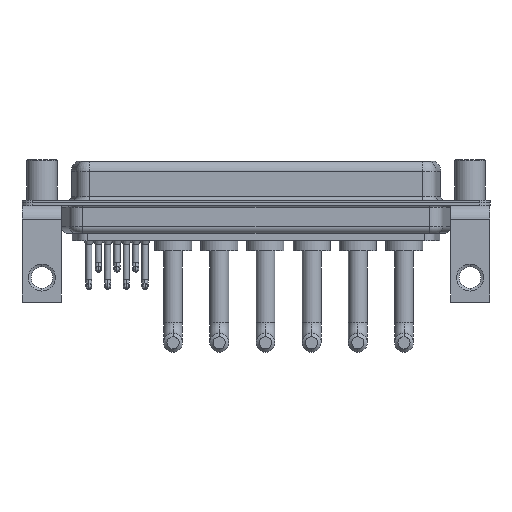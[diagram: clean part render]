
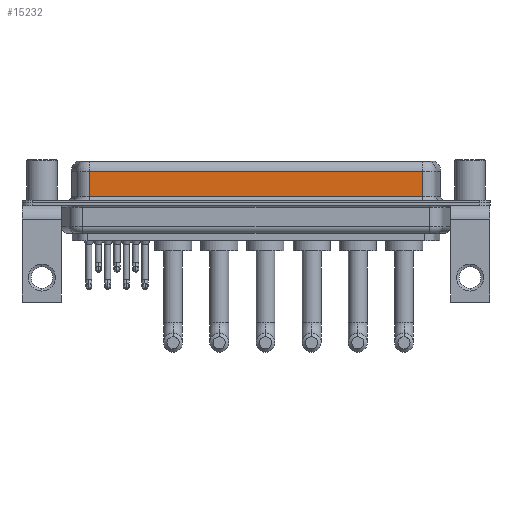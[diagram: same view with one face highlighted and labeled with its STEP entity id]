
A CAD part, front view. The second image highlights one B-rep face of the part: STEP entity #15232.
In plain terms, the highlighted planar face has unit normal (0, -1, 0).
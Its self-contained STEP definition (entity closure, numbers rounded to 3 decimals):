
#942 = CARTESIAN_POINT ( 'NONE',  ( 56.462, -3.95, 4.65 ) ) ;
#2173 = PLANE ( 'NONE',  #18245 ) ;
#3908 = CARTESIAN_POINT ( 'NONE',  ( 56.462, -3.95, 0.9 ) ) ;
#4089 = DIRECTION ( 'NONE',  ( 0., 0., 1. ) ) ;
#4454 = ORIENTED_EDGE ( 'NONE', *, *, #7155, .T. ) ;
#5026 = EDGE_CURVE ( 'NONE', #16293, #19661, #13982, .T. ) ;
#5248 = VECTOR ( 'NONE', #10387, 1000. ) ;
#5334 = CARTESIAN_POINT ( 'NONE',  ( 7.038, -3.95, 0.9 ) ) ;
#5919 = CARTESIAN_POINT ( 'NONE',  ( 56.462, -3.95, 6.4 ) ) ;
#5995 = CARTESIAN_POINT ( 'NONE',  ( 56.462, -3.95, 4.65 ) ) ;
#6094 = EDGE_LOOP ( 'NONE', ( #18858, #7365, #4454, #16967 ) ) ;
#6984 = VERTEX_POINT ( 'NONE', #9303 ) ;
#7155 = EDGE_CURVE ( 'NONE', #6984, #17763, #14881, .T. ) ;
#7365 = ORIENTED_EDGE ( 'NONE', *, *, #20162, .T. ) ;
#8211 = DIRECTION ( 'NONE',  ( 0., 0., -1. ) ) ;
#8445 = CARTESIAN_POINT ( 'NONE',  ( 56.462, -3.95, 6.4 ) ) ;
#8944 = EDGE_CURVE ( 'NONE', #17763, #19661, #20007, .T. ) ;
#9303 = CARTESIAN_POINT ( 'NONE',  ( 7.038, -3.95, 4.65 ) ) ;
#10387 = DIRECTION ( 'NONE',  ( 1., 0., 0. ) ) ;
#12153 = DIRECTION ( 'NONE',  ( 0., 1., 0. ) ) ;
#12254 = DIRECTION ( 'NONE',  ( -1., 0., 0. ) ) ;
#12968 = VECTOR ( 'NONE', #8211, 1000. ) ;
#13416 = CARTESIAN_POINT ( 'NONE',  ( 7.038, -3.95, 6.4 ) ) ;
#13982 = LINE ( 'NONE', #5919, #15748 ) ;
#14648 = VECTOR ( 'NONE', #12254, 1000. ) ;
#14881 = LINE ( 'NONE', #13416, #12968 ) ;
#15232 = ADVANCED_FACE ( 'NONE', ( #18170 ), #2173, .F. ) ;
#15748 = VECTOR ( 'NONE', #20321, 1000. ) ;
#16293 = VERTEX_POINT ( 'NONE', #942 ) ;
#16967 = ORIENTED_EDGE ( 'NONE', *, *, #8944, .T. ) ;
#17763 = VERTEX_POINT ( 'NONE', #5334 ) ;
#18170 = FACE_OUTER_BOUND ( 'NONE', #6094, .T. ) ;
#18245 = AXIS2_PLACEMENT_3D ( 'NONE', #8445, #12153, #4089 ) ;
#18640 = CARTESIAN_POINT ( 'NONE',  ( 56.462, -3.95, 0.9 ) ) ;
#18858 = ORIENTED_EDGE ( 'NONE', *, *, #5026, .F. ) ;
#19661 = VERTEX_POINT ( 'NONE', #18640 ) ;
#20007 = LINE ( 'NONE', #3908, #5248 ) ;
#20162 = EDGE_CURVE ( 'NONE', #16293, #6984, #20516, .T. ) ;
#20321 = DIRECTION ( 'NONE',  ( 0., 0., -1. ) ) ;
#20516 = LINE ( 'NONE', #5995, #14648 ) ;
